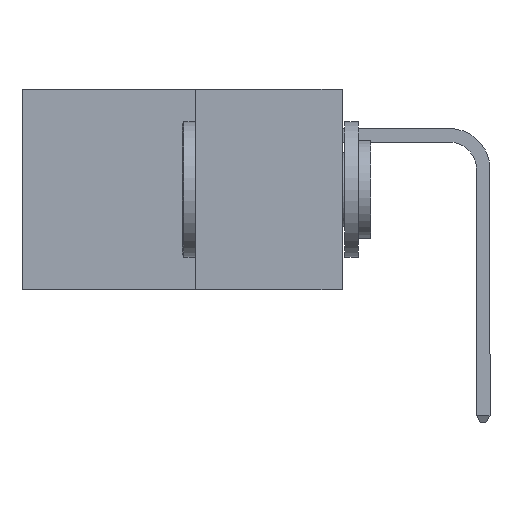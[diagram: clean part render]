
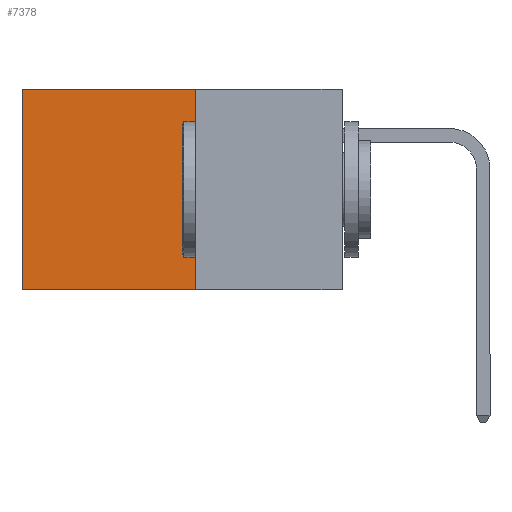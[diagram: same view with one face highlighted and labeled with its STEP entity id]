
A CAD part, left-side view. The second image highlights one B-rep face of the part: STEP entity #7378.
In plain terms, the highlighted planar face has unit normal (-1, 0, 0).
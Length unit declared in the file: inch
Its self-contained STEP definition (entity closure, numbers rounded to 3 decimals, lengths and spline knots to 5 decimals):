
#258 = CARTESIAN_POINT ( 'NONE',  ( 0.277, 0.27, 0. ) ) ;
#337 = DIRECTION ( 'NONE',  ( 0., 0., -1. ) ) ;
#729 = CARTESIAN_POINT ( 'NONE',  ( 0.277, 0.27, -0.37 ) ) ;
#768 = CARTESIAN_POINT ( 'NONE',  ( 0.277, 0.27, 0. ) ) ;
#812 = EDGE_CURVE ( 'NONE', #5783, #9296, #1784, .T. ) ;
#1431 = DIRECTION ( 'NONE',  ( 0., 0., -1. ) ) ;
#1478 = DIRECTION ( 'NONE',  ( 0., 1., 0. ) ) ;
#1497 = VECTOR ( 'NONE', #337, 39.37008 ) ;
#1723 = EDGE_CURVE ( 'NONE', #8423, #7572, #5897, .T. ) ;
#1784 = LINE ( 'NONE', #729, #1497 ) ;
#2612 = CARTESIAN_POINT ( 'NONE',  ( 0.277, 0.27, -0.37 ) ) ;
#2971 = ORIENTED_EDGE ( 'NONE', *, *, #4042, .F. ) ;
#2978 = EDGE_CURVE ( 'NONE', #5783, #8423, #7497, .T. ) ;
#3200 = VECTOR ( 'NONE', #1478, 39.37008 ) ;
#3568 = VECTOR ( 'NONE', #8776, 39.37008 ) ;
#3998 = AXIS2_PLACEMENT_3D ( 'NONE', #7877, #7495, #6278 ) ;
#4042 = EDGE_CURVE ( 'NONE', #9296, #7572, #9825, .T. ) ;
#4362 = CARTESIAN_POINT ( 'NONE',  ( 0.277, 0.59, -0.37 ) ) ;
#4872 = CARTESIAN_POINT ( 'NONE',  ( 0.277, 0.59, -0.37 ) ) ;
#5087 = EDGE_LOOP ( 'NONE', ( #7024, #2971, #7270, #9532 ) ) ;
#5783 = VERTEX_POINT ( 'NONE', #258 ) ;
#5897 = LINE ( 'NONE', #4362, #9745 ) ;
#6278 = DIRECTION ( 'NONE',  ( 0., 0., -1. ) ) ;
#7024 = ORIENTED_EDGE ( 'NONE', *, *, #1723, .T. ) ;
#7199 = CARTESIAN_POINT ( 'NONE',  ( 0.277, 0.59, 0. ) ) ;
#7270 = ORIENTED_EDGE ( 'NONE', *, *, #812, .F. ) ;
#7378 = ADVANCED_FACE ( 'NONE', ( #8915 ), #7618, .F. ) ;
#7495 = DIRECTION ( 'NONE',  ( 1., 0., 0. ) ) ;
#7497 = LINE ( 'NONE', #768, #3200 ) ;
#7572 = VERTEX_POINT ( 'NONE', #4872 ) ;
#7618 = PLANE ( 'NONE',  #3998 ) ;
#7877 = CARTESIAN_POINT ( 'NONE',  ( 0.277, 0.27, -0.37 ) ) ;
#8423 = VERTEX_POINT ( 'NONE', #7199 ) ;
#8513 = CARTESIAN_POINT ( 'NONE',  ( 0.277, 0.27, -0.37 ) ) ;
#8776 = DIRECTION ( 'NONE',  ( 0., 1., 0. ) ) ;
#8915 = FACE_OUTER_BOUND ( 'NONE', #5087, .T. ) ;
#9296 = VERTEX_POINT ( 'NONE', #2612 ) ;
#9532 = ORIENTED_EDGE ( 'NONE', *, *, #2978, .T. ) ;
#9745 = VECTOR ( 'NONE', #1431, 39.37008 ) ;
#9825 = LINE ( 'NONE', #8513, #3568 ) ;
